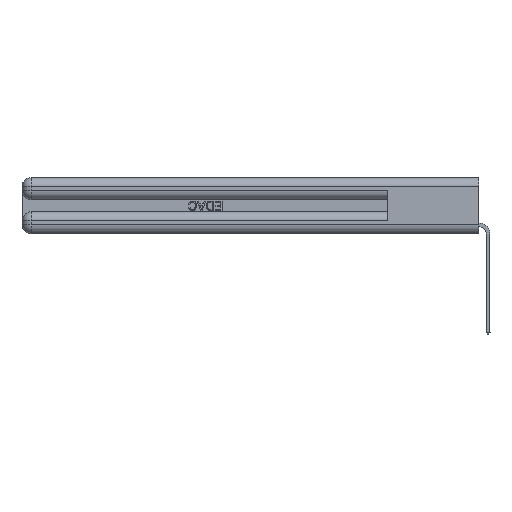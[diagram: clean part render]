
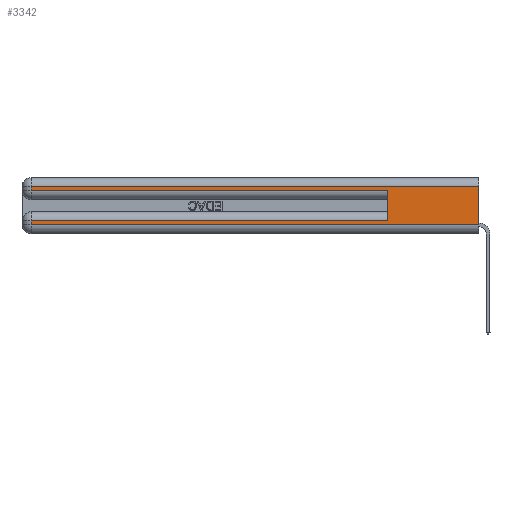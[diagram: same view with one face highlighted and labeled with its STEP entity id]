
A CAD part, left-side view. The second image highlights one B-rep face of the part: STEP entity #3342.
In plain terms, the highlighted planar face has unit normal (-1, 0, 0).
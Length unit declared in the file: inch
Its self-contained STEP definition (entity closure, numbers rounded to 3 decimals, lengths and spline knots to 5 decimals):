
#359 = EDGE_CURVE ( 'NONE', #26731, #23188, #22798, .T. ) ;
#376 = VECTOR ( 'NONE', #7824, 39.37008 ) ;
#450 = LINE ( 'NONE', #16059, #11011 ) ;
#1039 = LINE ( 'NONE', #24834, #376 ) ;
#1391 = ORIENTED_EDGE ( 'NONE', *, *, #20538, .T. ) ;
#1532 = CARTESIAN_POINT ( 'NONE',  ( 0., 2.94, 0.06 ) ) ;
#1764 = ORIENTED_EDGE ( 'NONE', *, *, #2474, .T. ) ;
#1825 = CARTESIAN_POINT ( 'NONE',  ( 0., 0., 0.06 ) ) ;
#2009 = DIRECTION ( 'NONE',  ( 1., 0., 0. ) ) ;
#2010 = VERTEX_POINT ( 'NONE', #20914 ) ;
#2474 = EDGE_CURVE ( 'NONE', #22992, #19368, #450, .T. ) ;
#2651 = AXIS2_PLACEMENT_3D ( 'NONE', #14682, #2009, #16850 ) ;
#2935 = ORIENTED_EDGE ( 'NONE', *, *, #14601, .F. ) ;
#3042 = ORIENTED_EDGE ( 'NONE', *, *, #22002, .T. ) ;
#3171 = LINE ( 'NONE', #1825, #13720 ) ;
#3342 = ADVANCED_FACE ( 'NONE', ( #19105 ), #25301, .F. ) ;
#3795 = ORIENTED_EDGE ( 'NONE', *, *, #6453, .F. ) ;
#4214 = EDGE_CURVE ( 'NONE', #23931, #23918, #21030, .T. ) ;
#4866 = ORIENTED_EDGE ( 'NONE', *, *, #12922, .T. ) ;
#5138 = CARTESIAN_POINT ( 'NONE',  ( 0., 2.94, 0.085 ) ) ;
#6286 = VECTOR ( 'NONE', #22021, 39.37008 ) ;
#6453 = EDGE_CURVE ( 'NONE', #23931, #2010, #11242, .T. ) ;
#7689 = VERTEX_POINT ( 'NONE', #19429 ) ;
#7757 = VECTOR ( 'NONE', #16449, 39.37008 ) ;
#7824 = DIRECTION ( 'NONE',  ( 0., 1., 0. ) ) ;
#8204 = CARTESIAN_POINT ( 'NONE',  ( 0., 0., 0.31 ) ) ;
#10234 = DIRECTION ( 'NONE',  ( 0., -1., 0. ) ) ;
#11011 = VECTOR ( 'NONE', #22472, 39.37008 ) ;
#11242 = LINE ( 'NONE', #17837, #6286 ) ;
#12128 = VECTOR ( 'NONE', #23912, 39.37008 ) ;
#12722 = CARTESIAN_POINT ( 'NONE',  ( 0., 0.6, 0.145 ) ) ;
#12922 = EDGE_CURVE ( 'NONE', #19368, #2010, #3171, .T. ) ;
#13371 = LINE ( 'NONE', #24920, #7757 ) ;
#13720 = VECTOR ( 'NONE', #10234, 39.37008 ) ;
#13799 = EDGE_LOOP ( 'NONE', ( #3795, #25986, #3042, #20193, #2935, #1391, #1764, #4866 ) ) ;
#13955 = VECTOR ( 'NONE', #14866, 39.37008 ) ;
#14601 = EDGE_CURVE ( 'NONE', #7689, #23188, #15304, .T. ) ;
#14682 = CARTESIAN_POINT ( 'NONE',  ( 0., 0., 0.37 ) ) ;
#14866 = DIRECTION ( 'NONE',  ( 0., 0., 1. ) ) ;
#15304 = LINE ( 'NONE', #12722, #13955 ) ;
#15369 = VECTOR ( 'NONE', #27215, 39.37008 ) ;
#16059 = CARTESIAN_POINT ( 'NONE',  ( 0., 2.94, 0.37 ) ) ;
#16449 = DIRECTION ( 'NONE',  ( 0., 0., -1. ) ) ;
#16850 = DIRECTION ( 'NONE',  ( 0., 0., -1. ) ) ;
#17600 = CARTESIAN_POINT ( 'NONE',  ( 0., 2.94, 0.285 ) ) ;
#17837 = CARTESIAN_POINT ( 'NONE',  ( 0., 0., 0.37 ) ) ;
#19105 = FACE_OUTER_BOUND ( 'NONE', #13799, .T. ) ;
#19368 = VERTEX_POINT ( 'NONE', #1532 ) ;
#19429 = CARTESIAN_POINT ( 'NONE',  ( 0., 0.6, 0.085 ) ) ;
#20193 = ORIENTED_EDGE ( 'NONE', *, *, #359, .T. ) ;
#20538 = EDGE_CURVE ( 'NONE', #7689, #22992, #1039, .T. ) ;
#20914 = CARTESIAN_POINT ( 'NONE',  ( 0., 0., 0.06 ) ) ;
#21030 = LINE ( 'NONE', #25097, #15369 ) ;
#22002 = EDGE_CURVE ( 'NONE', #23918, #26731, #13371, .T. ) ;
#22021 = DIRECTION ( 'NONE',  ( 0., 0., -1. ) ) ;
#22472 = DIRECTION ( 'NONE',  ( 0., 0., -1. ) ) ;
#22798 = LINE ( 'NONE', #24103, #12128 ) ;
#22980 = CARTESIAN_POINT ( 'NONE',  ( 0., 2.94, 0.31 ) ) ;
#22992 = VERTEX_POINT ( 'NONE', #5138 ) ;
#23188 = VERTEX_POINT ( 'NONE', #24778 ) ;
#23912 = DIRECTION ( 'NONE',  ( 0., -1., 0. ) ) ;
#23918 = VERTEX_POINT ( 'NONE', #22980 ) ;
#23931 = VERTEX_POINT ( 'NONE', #8204 ) ;
#24103 = CARTESIAN_POINT ( 'NONE',  ( 0., 0., 0.285 ) ) ;
#24778 = CARTESIAN_POINT ( 'NONE',  ( 0., 0.6, 0.285 ) ) ;
#24834 = CARTESIAN_POINT ( 'NONE',  ( 0., 0., 0.085 ) ) ;
#24920 = CARTESIAN_POINT ( 'NONE',  ( 0., 2.94, 0.37 ) ) ;
#25097 = CARTESIAN_POINT ( 'NONE',  ( 0., 0., 0.31 ) ) ;
#25301 = PLANE ( 'NONE',  #2651 ) ;
#25986 = ORIENTED_EDGE ( 'NONE', *, *, #4214, .T. ) ;
#26731 = VERTEX_POINT ( 'NONE', #17600 ) ;
#27215 = DIRECTION ( 'NONE',  ( 0., 1., 0. ) ) ;
